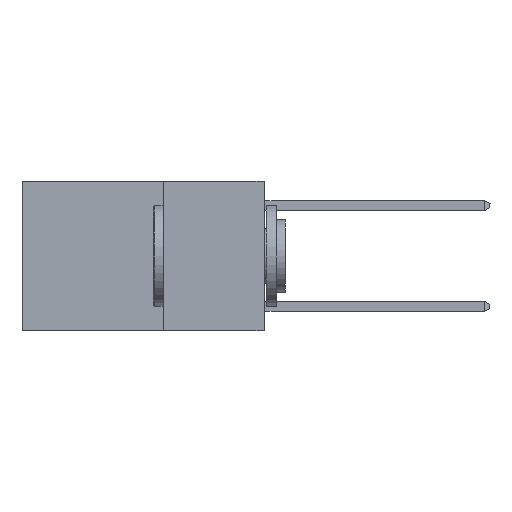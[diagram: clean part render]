
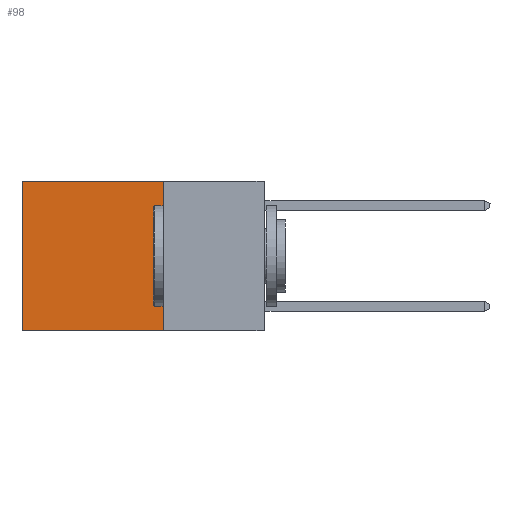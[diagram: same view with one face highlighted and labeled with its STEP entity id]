
A CAD part, left-side view. The second image highlights one B-rep face of the part: STEP entity #98.
In plain terms, the highlighted planar face has unit normal (-1, 0, 0).
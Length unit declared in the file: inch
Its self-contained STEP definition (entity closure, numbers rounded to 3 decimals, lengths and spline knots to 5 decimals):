
#98 = ADVANCED_FACE ( 'NONE', ( #5219 ), #4550, .F. ) ;
#345 = VECTOR ( 'NONE', #4805, 39.37008 ) ;
#730 = LINE ( 'NONE', #8515, #1575 ) ;
#1037 = DIRECTION ( 'NONE',  ( 0., 0., -1. ) ) ;
#1131 = DIRECTION ( 'NONE',  ( 0., 1., 0. ) ) ;
#1222 = ORIENTED_EDGE ( 'NONE', *, *, #8193, .T. ) ;
#1368 = EDGE_LOOP ( 'NONE', ( #1387, #4549, #2226, #1222 ) ) ;
#1387 = ORIENTED_EDGE ( 'NONE', *, *, #10066, .T. ) ;
#1575 = VECTOR ( 'NONE', #9344, 39.37008 ) ;
#2090 = CARTESIAN_POINT ( 'NONE',  ( 0.2625, 0.6, 0. ) ) ;
#2226 = ORIENTED_EDGE ( 'NONE', *, *, #7924, .F. ) ;
#2722 = CARTESIAN_POINT ( 'NONE',  ( 0.2625, 0.25, -0.37 ) ) ;
#2756 = DIRECTION ( 'NONE',  ( 0., 0., -1. ) ) ;
#3219 = CARTESIAN_POINT ( 'NONE',  ( 0.2625, 0.6, 0. ) ) ;
#3479 = VERTEX_POINT ( 'NONE', #2090 ) ;
#3685 = AXIS2_PLACEMENT_3D ( 'NONE', #10509, #8824, #1037 ) ;
#4252 = CARTESIAN_POINT ( 'NONE',  ( 0.2625, 0.25, -0.37 ) ) ;
#4549 = ORIENTED_EDGE ( 'NONE', *, *, #9887, .F. ) ;
#4550 = PLANE ( 'NONE',  #3685 ) ;
#4805 = DIRECTION ( 'NONE',  ( 0., 0., -1. ) ) ;
#4821 = CARTESIAN_POINT ( 'NONE',  ( 0.2625, 0.25, 0. ) ) ;
#5219 = FACE_OUTER_BOUND ( 'NONE', #1368, .T. ) ;
#5710 = CARTESIAN_POINT ( 'NONE',  ( 0.2625, 0.6, -0.37 ) ) ;
#6131 = LINE ( 'NONE', #2722, #6168 ) ;
#6168 = VECTOR ( 'NONE', #1131, 39.37008 ) ;
#7778 = LINE ( 'NONE', #8588, #7895 ) ;
#7895 = VECTOR ( 'NONE', #2756, 39.37008 ) ;
#7924 = EDGE_CURVE ( 'NONE', #9626, #8684, #7778, .T. ) ;
#8193 = EDGE_CURVE ( 'NONE', #9626, #3479, #730, .T. ) ;
#8515 = CARTESIAN_POINT ( 'NONE',  ( 0.2625, 0.25, 0. ) ) ;
#8588 = CARTESIAN_POINT ( 'NONE',  ( 0.2625, 0.25, 0. ) ) ;
#8684 = VERTEX_POINT ( 'NONE', #4252 ) ;
#8824 = DIRECTION ( 'NONE',  ( 1., 0., 0. ) ) ;
#9344 = DIRECTION ( 'NONE',  ( 0., 1., 0. ) ) ;
#9626 = VERTEX_POINT ( 'NONE', #4821 ) ;
#9630 = VERTEX_POINT ( 'NONE', #5710 ) ;
#9887 = EDGE_CURVE ( 'NONE', #8684, #9630, #6131, .T. ) ;
#10066 = EDGE_CURVE ( 'NONE', #3479, #9630, #10656, .T. ) ;
#10509 = CARTESIAN_POINT ( 'NONE',  ( 0.2625, 0.25, 0. ) ) ;
#10656 = LINE ( 'NONE', #3219, #345 ) ;
